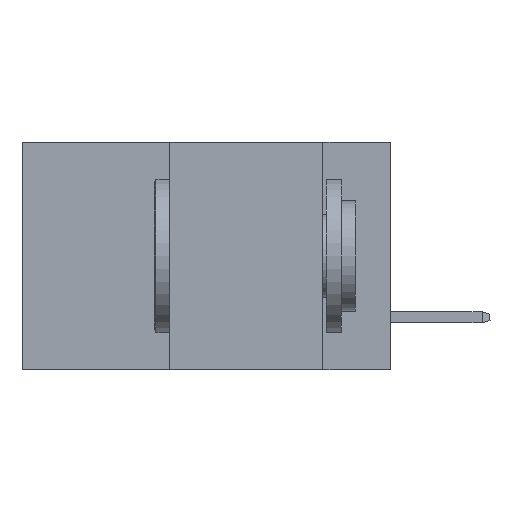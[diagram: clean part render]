
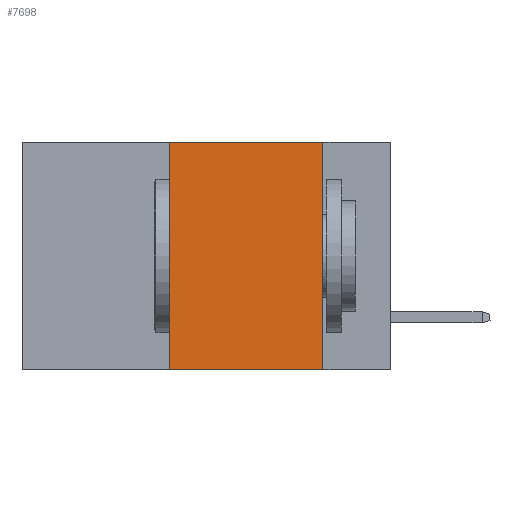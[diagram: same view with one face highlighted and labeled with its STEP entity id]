
A CAD part, left-side view. The second image highlights one B-rep face of the part: STEP entity #7698.
In plain terms, the highlighted planar face has unit normal (-1, 0, 0).
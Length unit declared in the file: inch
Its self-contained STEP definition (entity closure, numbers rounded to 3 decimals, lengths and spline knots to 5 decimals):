
#234 = LINE ( 'NONE', #9596, #10571 ) ;
#304 = LINE ( 'NONE', #2216, #9608 ) ;
#514 = LINE ( 'NONE', #3954, #5600 ) ;
#573 = FACE_OUTER_BOUND ( 'NONE', #3469, .T. ) ;
#721 = CARTESIAN_POINT ( 'NONE',  ( 0., 0.36, 0. ) ) ;
#742 = DIRECTION ( 'NONE',  ( 0., 0., 1. ) ) ;
#891 = DIRECTION ( 'NONE',  ( 1., 0., 0. ) ) ;
#1719 = DIRECTION ( 'NONE',  ( 0., 0., -1. ) ) ;
#1753 = EDGE_CURVE ( 'NONE', #7680, #1821, #514, .T. ) ;
#1754 = ORIENTED_EDGE ( 'NONE', *, *, #1753, .T. ) ;
#1821 = VERTEX_POINT ( 'NONE', #6305 ) ;
#2216 = CARTESIAN_POINT ( 'NONE',  ( 0., 0.6, 0. ) ) ;
#2819 = EDGE_CURVE ( 'NONE', #9857, #1821, #234, .T. ) ;
#2908 = DIRECTION ( 'NONE',  ( 0., 0., -1. ) ) ;
#3063 = DIRECTION ( 'NONE',  ( 0., -1., 0. ) ) ;
#3371 = CARTESIAN_POINT ( 'NONE',  ( 0., 0.6, 0. ) ) ;
#3469 = EDGE_LOOP ( 'NONE', ( #3955, #10153, #9060, #1754 ) ) ;
#3954 = CARTESIAN_POINT ( 'NONE',  ( 0., 0.6, -0.37 ) ) ;
#3955 = ORIENTED_EDGE ( 'NONE', *, *, #2819, .F. ) ;
#4521 = CARTESIAN_POINT ( 'NONE',  ( 0., 0.11, 0. ) ) ;
#5600 = VECTOR ( 'NONE', #9021, 39.37008 ) ;
#5850 = CARTESIAN_POINT ( 'NONE',  ( 0., 0.36, -0.37 ) ) ;
#6003 = AXIS2_PLACEMENT_3D ( 'NONE', #3371, #891, #1719 ) ;
#6305 = CARTESIAN_POINT ( 'NONE',  ( 0., 0.11, -0.37 ) ) ;
#6930 = LINE ( 'NONE', #10126, #8985 ) ;
#7328 = VERTEX_POINT ( 'NONE', #721 ) ;
#7680 = VERTEX_POINT ( 'NONE', #5850 ) ;
#7698 = ADVANCED_FACE ( 'NONE', ( #573 ), #8270, .F. ) ;
#7787 = EDGE_CURVE ( 'NONE', #7680, #7328, #6930, .T. ) ;
#8230 = EDGE_CURVE ( 'NONE', #7328, #9857, #304, .T. ) ;
#8270 = PLANE ( 'NONE',  #6003 ) ;
#8985 = VECTOR ( 'NONE', #742, 39.37008 ) ;
#9021 = DIRECTION ( 'NONE',  ( 0., -1., 0. ) ) ;
#9060 = ORIENTED_EDGE ( 'NONE', *, *, #7787, .F. ) ;
#9596 = CARTESIAN_POINT ( 'NONE',  ( 0., 0.11, 0. ) ) ;
#9608 = VECTOR ( 'NONE', #3063, 39.37008 ) ;
#9857 = VERTEX_POINT ( 'NONE', #4521 ) ;
#10126 = CARTESIAN_POINT ( 'NONE',  ( 0., 0.36, 0. ) ) ;
#10153 = ORIENTED_EDGE ( 'NONE', *, *, #8230, .F. ) ;
#10571 = VECTOR ( 'NONE', #2908, 39.37008 ) ;
